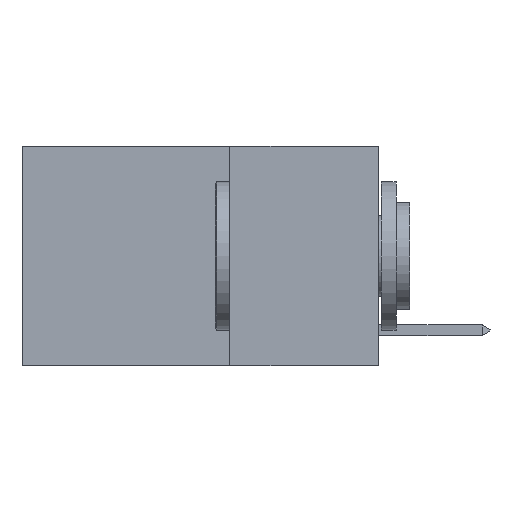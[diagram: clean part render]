
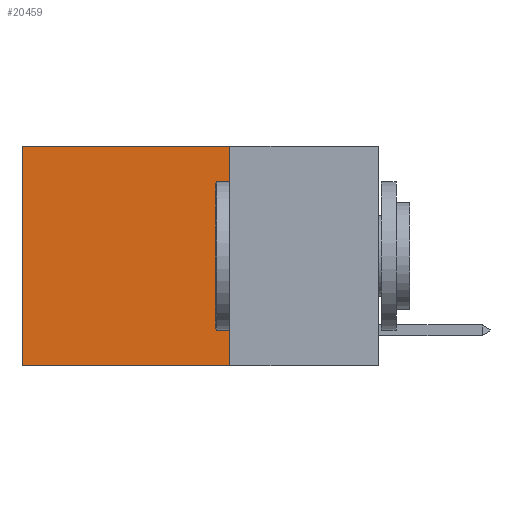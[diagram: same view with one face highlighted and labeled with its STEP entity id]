
A CAD part, left-side view. The second image highlights one B-rep face of the part: STEP entity #20459.
In plain terms, the highlighted planar face has unit normal (-1, 0, 0).
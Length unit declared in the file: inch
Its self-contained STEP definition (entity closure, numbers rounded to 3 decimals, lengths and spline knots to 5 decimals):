
#44 = DIRECTION ( 'NONE',  ( 0., 0., -1. ) ) ;
#502 = LINE ( 'NONE', #5878, #24946 ) ;
#2381 = VECTOR ( 'NONE', #3823, 39.37008 ) ;
#2382 = AXIS2_PLACEMENT_3D ( 'NONE', #16125, #8242, #44 ) ;
#3412 = VERTEX_POINT ( 'NONE', #23856 ) ;
#3823 = DIRECTION ( 'NONE',  ( 0., 1., 0. ) ) ;
#4307 = DIRECTION ( 'NONE',  ( 0., 1., 0. ) ) ;
#5559 = VERTEX_POINT ( 'NONE', #6450 ) ;
#5606 = EDGE_CURVE ( 'NONE', #8704, #5559, #24389, .T. ) ;
#5878 = CARTESIAN_POINT ( 'NONE',  ( 0.2625, 0.25, -0.37 ) ) ;
#6450 = CARTESIAN_POINT ( 'NONE',  ( 0.2625, 0.25, -0.37 ) ) ;
#6518 = LINE ( 'NONE', #22501, #17842 ) ;
#6796 = ORIENTED_EDGE ( 'NONE', *, *, #5606, .F. ) ;
#7314 = LINE ( 'NONE', #15342, #2381 ) ;
#8179 = EDGE_CURVE ( 'NONE', #8704, #12744, #7314, .T. ) ;
#8242 = DIRECTION ( 'NONE',  ( 1., 0., 0. ) ) ;
#8704 = VERTEX_POINT ( 'NONE', #19865 ) ;
#9040 = ORIENTED_EDGE ( 'NONE', *, *, #8179, .T. ) ;
#12109 = DIRECTION ( 'NONE',  ( 0., 0., -1. ) ) ;
#12744 = VERTEX_POINT ( 'NONE', #21661 ) ;
#13007 = ORIENTED_EDGE ( 'NONE', *, *, #20635, .T. ) ;
#15342 = CARTESIAN_POINT ( 'NONE',  ( 0.2625, 0.25, 0. ) ) ;
#16125 = CARTESIAN_POINT ( 'NONE',  ( 0.2625, 0.25, 0. ) ) ;
#16188 = CARTESIAN_POINT ( 'NONE',  ( 0.2625, 0.25, 0. ) ) ;
#16262 = EDGE_CURVE ( 'NONE', #5559, #3412, #502, .T. ) ;
#17842 = VECTOR ( 'NONE', #18707, 39.37008 ) ;
#18707 = DIRECTION ( 'NONE',  ( 0., 0., -1. ) ) ;
#19325 = VECTOR ( 'NONE', #12109, 39.37008 ) ;
#19865 = CARTESIAN_POINT ( 'NONE',  ( 0.2625, 0.25, 0. ) ) ;
#20459 = ADVANCED_FACE ( 'NONE', ( #25778 ), #24331, .F. ) ;
#20635 = EDGE_CURVE ( 'NONE', #12744, #3412, #6518, .T. ) ;
#21661 = CARTESIAN_POINT ( 'NONE',  ( 0.2625, 0.6, 0. ) ) ;
#22501 = CARTESIAN_POINT ( 'NONE',  ( 0.2625, 0.6, 0. ) ) ;
#22766 = EDGE_LOOP ( 'NONE', ( #13007, #25093, #6796, #9040 ) ) ;
#23856 = CARTESIAN_POINT ( 'NONE',  ( 0.2625, 0.6, -0.37 ) ) ;
#24331 = PLANE ( 'NONE',  #2382 ) ;
#24389 = LINE ( 'NONE', #16188, #19325 ) ;
#24946 = VECTOR ( 'NONE', #4307, 39.37008 ) ;
#25093 = ORIENTED_EDGE ( 'NONE', *, *, #16262, .F. ) ;
#25778 = FACE_OUTER_BOUND ( 'NONE', #22766, .T. ) ;
